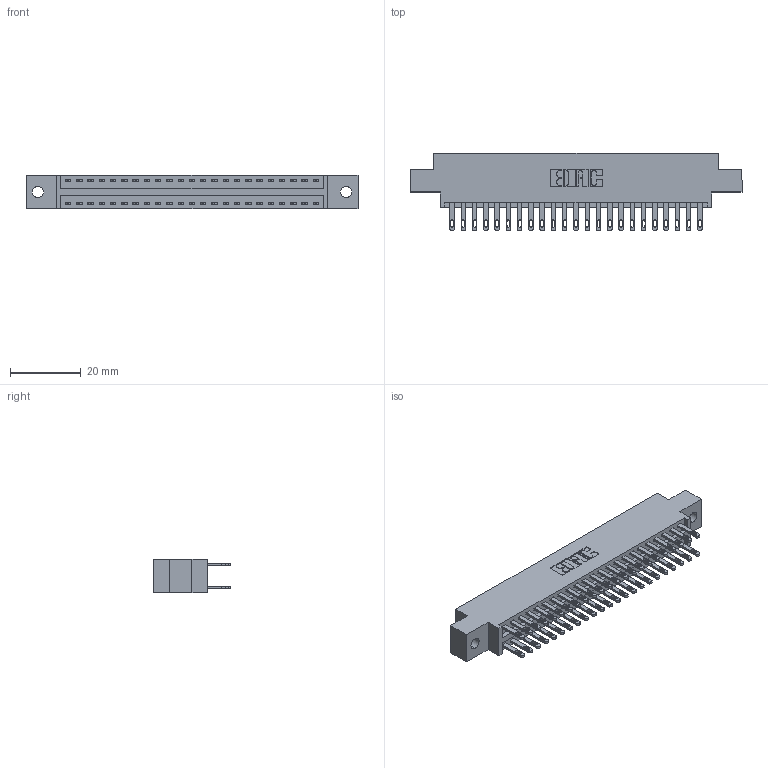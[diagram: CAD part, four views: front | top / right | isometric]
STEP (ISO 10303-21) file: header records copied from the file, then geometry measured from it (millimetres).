
FILE_DESCRIPTION (( 'STEP AP203' ), '1' );
FILE_NAME ('346-046-500-802.STEP', '2018-08-25T04:33:32', ( '' ), ( '' ), 'SwSTEP 2.0', 'SolidWorks 2016', '' );
FILE_SCHEMA (( 'CONFIG_CONTROL_DESIGN' ));
Length unit declared in the file: inch
Products named in the file (3): 346-046-500-802; 346 Part_0.170 Offset - 0.128 Dia; 345-292-001_345-293-100
Assembly tree (47 placements, depth 2):
  346-046-500-802
    346 Part_0.170 Offset - 0.128 Dia
    345-292-001_345-293-100  x46
Bounding box: 93.6 x 21.84 x 9.4 mm (x, y, z)
Volume: 8928.8 mm3; surface area: 12366.4 mm2
Topology: 47 solids, 47 shells, 2334 faces, 7103 edges, 4734 vertices
Faces by surface type: plane 1414, cylinder 920
Entity records: 17633 total; most frequent: CARTESIAN_POINT 2932, ORIENTED_EDGE 2866, DIRECTION 2637, EDGE_CURVE 1433, VECTOR 1205, LINE 1205, VERTEX_POINT 954, AXIS2_PLACEMENT_3D 716
